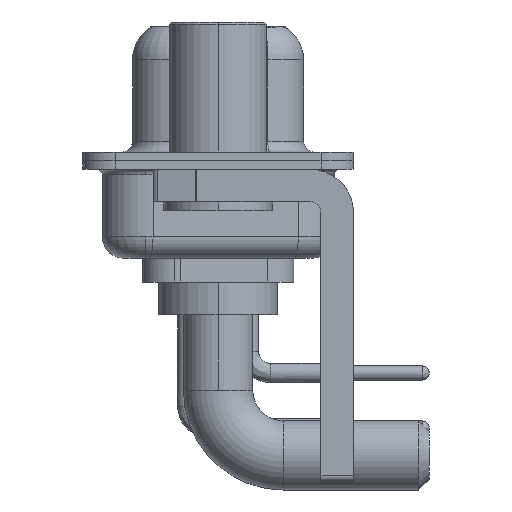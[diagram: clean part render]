
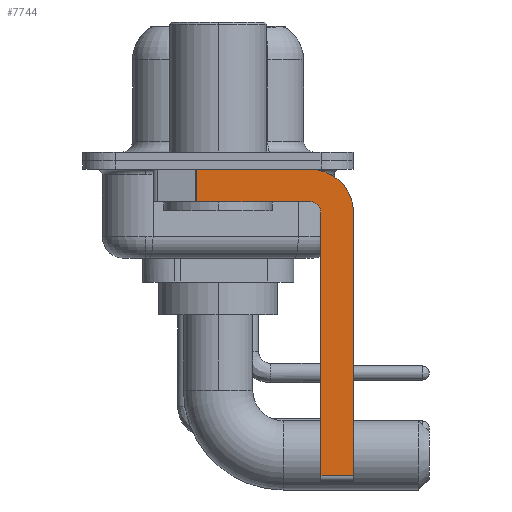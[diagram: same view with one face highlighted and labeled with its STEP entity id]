
A CAD part, left-side view. The second image highlights one B-rep face of the part: STEP entity #7744.
In plain terms, the highlighted planar face has unit normal (-1, 0, 0).
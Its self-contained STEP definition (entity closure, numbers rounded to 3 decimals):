
#301 = CARTESIAN_POINT ( 'NONE',  ( -2.9, -4.25, -1.9 ) ) ;
#2197 = AXIS2_PLACEMENT_3D ( 'NONE', #2914, #11553, #2803 ) ;
#2278 = EDGE_CURVE ( 'NONE', #17712, #15524, #2846, .T. ) ;
#2558 = VERTEX_POINT ( 'NONE', #18334 ) ;
#2803 = DIRECTION ( 'NONE',  ( 0., 0., -1. ) ) ;
#2846 = LINE ( 'NONE', #19166, #20012 ) ;
#2914 = CARTESIAN_POINT ( 'NONE',  ( -2.9, -4.25, -2.4 ) ) ;
#3081 = CARTESIAN_POINT ( 'NONE',  ( -2.9, -6.25, -2.4 ) ) ;
#3293 = CARTESIAN_POINT ( 'NONE',  ( -2.9, -4.75, -2.4 ) ) ;
#3415 = EDGE_CURVE ( 'NONE', #4111, #4124, #22748, .T. ) ;
#3522 = VECTOR ( 'NONE', #6380, 1000. ) ;
#3741 = DIRECTION ( 'NONE',  ( 0., 0., 1. ) ) ;
#4111 = VERTEX_POINT ( 'NONE', #21119 ) ;
#4124 = VERTEX_POINT ( 'NONE', #17929 ) ;
#4133 = ORIENTED_EDGE ( 'NONE', *, *, #18154, .F. ) ;
#4279 = DIRECTION ( 'NONE',  ( 1., 0., 0. ) ) ;
#4443 = VERTEX_POINT ( 'NONE', #6061 ) ;
#6040 = VERTEX_POINT ( 'NONE', #3293 ) ;
#6061 = CARTESIAN_POINT ( 'NONE',  ( -2.9, -4.25, -1.9 ) ) ;
#6380 = DIRECTION ( 'NONE',  ( 0., 0., -1. ) ) ;
#6501 = LINE ( 'NONE', #3081, #3522 ) ;
#6614 = EDGE_CURVE ( 'NONE', #4443, #2558, #16496, .T. ) ;
#7676 = DIRECTION ( 'NONE',  ( 0., 0., -1. ) ) ;
#7744 = ADVANCED_FACE ( 'NONE', ( #22442 ), #9880, .F. ) ;
#8255 = DIRECTION ( 'NONE',  ( 0., 0., 1. ) ) ;
#8391 = DIRECTION ( 'NONE',  ( 0., -1., 0. ) ) ;
#8550 = EDGE_CURVE ( 'NONE', #8887, #2558, #9691, .T. ) ;
#8834 = AXIS2_PLACEMENT_3D ( 'NONE', #15718, #11934, #8255 ) ;
#8887 = VERTEX_POINT ( 'NONE', #12840 ) ;
#9218 = VECTOR ( 'NONE', #12478, 1000. ) ;
#9691 = LINE ( 'NONE', #22242, #17273 ) ;
#9880 = PLANE ( 'NONE',  #2197 ) ;
#9894 = AXIS2_PLACEMENT_3D ( 'NONE', #16573, #4279, #18711 ) ;
#11553 = DIRECTION ( 'NONE',  ( 1., 0., 0. ) ) ;
#11755 = LINE ( 'NONE', #17092, #15927 ) ;
#11934 = DIRECTION ( 'NONE',  ( -1., 0., 0. ) ) ;
#12230 = CIRCLE ( 'NONE', #8834, 0.5 ) ;
#12478 = DIRECTION ( 'NONE',  ( 0., 1., 0. ) ) ;
#12840 = CARTESIAN_POINT ( 'NONE',  ( -2.9, 0.978, -0.4 ) ) ;
#12843 = LINE ( 'NONE', #19949, #19817 ) ;
#13032 = ORIENTED_EDGE ( 'NONE', *, *, #22491, .F. ) ;
#15022 = ORIENTED_EDGE ( 'NONE', *, *, #8550, .T. ) ;
#15524 = VERTEX_POINT ( 'NONE', #18592 ) ;
#15584 = EDGE_CURVE ( 'NONE', #4124, #15524, #6501, .T. ) ;
#15718 = CARTESIAN_POINT ( 'NONE',  ( -2.9, -4.25, -2.4 ) ) ;
#15927 = VECTOR ( 'NONE', #16969, 1000. ) ;
#16496 = LINE ( 'NONE', #301, #9218 ) ;
#16573 = CARTESIAN_POINT ( 'NONE',  ( -2.9, -4.25, -2.4 ) ) ;
#16969 = DIRECTION ( 'NONE',  ( 0., -1., 0. ) ) ;
#17092 = CARTESIAN_POINT ( 'NONE',  ( -2.9, 3., -0.4 ) ) ;
#17273 = VECTOR ( 'NONE', #7676, 1000. ) ;
#17712 = VERTEX_POINT ( 'NONE', #22126 ) ;
#17929 = CARTESIAN_POINT ( 'NONE',  ( -2.9, -6.25, -2.4 ) ) ;
#18154 = EDGE_CURVE ( 'NONE', #6040, #4443, #12230, .T. ) ;
#18334 = CARTESIAN_POINT ( 'NONE',  ( -2.9, 0.978, -1.9 ) ) ;
#18459 = ORIENTED_EDGE ( 'NONE', *, *, #6614, .F. ) ;
#18592 = CARTESIAN_POINT ( 'NONE',  ( -2.9, -6.25, -14.55 ) ) ;
#18620 = EDGE_CURVE ( 'NONE', #17712, #6040, #12843, .T. ) ;
#18711 = DIRECTION ( 'NONE',  ( 0., 0., -1. ) ) ;
#19166 = CARTESIAN_POINT ( 'NONE',  ( -2.9, -4.25, -14.55 ) ) ;
#19817 = VECTOR ( 'NONE', #3741, 1000. ) ;
#19949 = CARTESIAN_POINT ( 'NONE',  ( -2.9, -4.75, -14.8 ) ) ;
#20012 = VECTOR ( 'NONE', #8391, 1000. ) ;
#20580 = EDGE_LOOP ( 'NONE', ( #13032, #15022, #18459, #4133, #21236, #21559, #21517, #22722 ) ) ;
#21119 = CARTESIAN_POINT ( 'NONE',  ( -2.9, -4.25, -0.4 ) ) ;
#21236 = ORIENTED_EDGE ( 'NONE', *, *, #18620, .F. ) ;
#21517 = ORIENTED_EDGE ( 'NONE', *, *, #15584, .F. ) ;
#21559 = ORIENTED_EDGE ( 'NONE', *, *, #2278, .T. ) ;
#22126 = CARTESIAN_POINT ( 'NONE',  ( -2.9, -4.75, -14.55 ) ) ;
#22242 = CARTESIAN_POINT ( 'NONE',  ( -2.9, 0.978, -1.9 ) ) ;
#22442 = FACE_OUTER_BOUND ( 'NONE', #20580, .T. ) ;
#22491 = EDGE_CURVE ( 'NONE', #8887, #4111, #11755, .T. ) ;
#22722 = ORIENTED_EDGE ( 'NONE', *, *, #3415, .F. ) ;
#22748 = CIRCLE ( 'NONE', #9894, 2. ) ;
